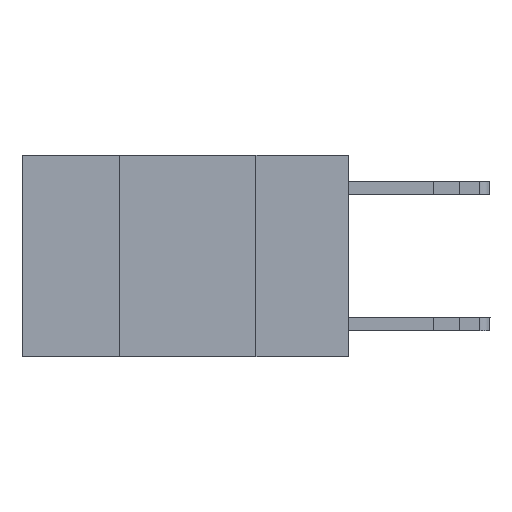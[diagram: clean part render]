
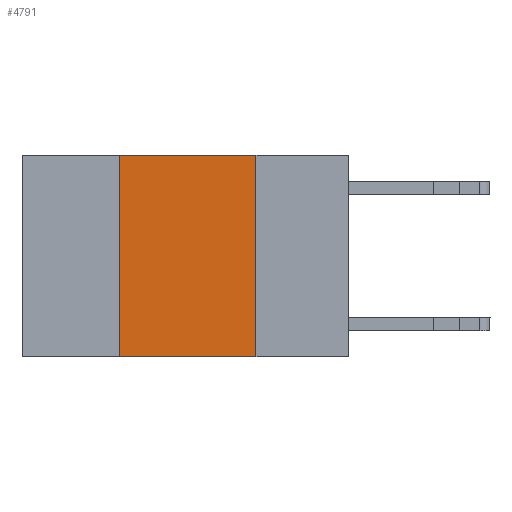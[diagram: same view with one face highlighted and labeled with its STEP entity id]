
A CAD part, left-side view. The second image highlights one B-rep face of the part: STEP entity #4791.
In plain terms, the highlighted planar face has unit normal (-1, 0, 0).
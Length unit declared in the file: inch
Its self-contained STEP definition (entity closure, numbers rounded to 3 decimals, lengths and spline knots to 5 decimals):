
#941 = VECTOR ( 'NONE', #6469, 39.37008 ) ;
#988 = DIRECTION ( 'NONE',  ( 1., 0., 0. ) ) ;
#1052 = LINE ( 'NONE', #8355, #4122 ) ;
#1350 = CARTESIAN_POINT ( 'NONE',  ( 0., 0.17, 0. ) ) ;
#1375 = ORIENTED_EDGE ( 'NONE', *, *, #9001, .T. ) ;
#1661 = LINE ( 'NONE', #10824, #4728 ) ;
#1981 = DIRECTION ( 'NONE',  ( 0., -1., 0. ) ) ;
#3002 = VERTEX_POINT ( 'NONE', #1350 ) ;
#3018 = ORIENTED_EDGE ( 'NONE', *, *, #3946, .F. ) ;
#3277 = VECTOR ( 'NONE', #4234, 39.37008 ) ;
#3498 = VERTEX_POINT ( 'NONE', #16098 ) ;
#3559 = AXIS2_PLACEMENT_3D ( 'NONE', #6138, #988, #9892 ) ;
#3635 = ORIENTED_EDGE ( 'NONE', *, *, #5650, .F. ) ;
#3685 = LINE ( 'NONE', #4189, #3277 ) ;
#3946 = EDGE_CURVE ( 'NONE', #3002, #3498, #1052, .T. ) ;
#4122 = VECTOR ( 'NONE', #10833, 39.37008 ) ;
#4189 = CARTESIAN_POINT ( 'NONE',  ( 0., 0.6, 0. ) ) ;
#4234 = DIRECTION ( 'NONE',  ( 0., -1., 0. ) ) ;
#4728 = VECTOR ( 'NONE', #1981, 39.37008 ) ;
#4791 = ADVANCED_FACE ( 'NONE', ( #7867 ), #7395, .F. ) ;
#5650 = EDGE_CURVE ( 'NONE', #8100, #6380, #11046, .T. ) ;
#6138 = CARTESIAN_POINT ( 'NONE',  ( 0., 0.6, 0. ) ) ;
#6380 = VERTEX_POINT ( 'NONE', #12698 ) ;
#6469 = DIRECTION ( 'NONE',  ( 0., 0., 1. ) ) ;
#6978 = EDGE_LOOP ( 'NONE', ( #3018, #12429, #3635, #1375 ) ) ;
#7395 = PLANE ( 'NONE',  #3559 ) ;
#7867 = FACE_OUTER_BOUND ( 'NONE', #6978, .T. ) ;
#8100 = VERTEX_POINT ( 'NONE', #14008 ) ;
#8355 = CARTESIAN_POINT ( 'NONE',  ( 0., 0.17, 0. ) ) ;
#9001 = EDGE_CURVE ( 'NONE', #8100, #3498, #1661, .T. ) ;
#9892 = DIRECTION ( 'NONE',  ( 0., 0., -1. ) ) ;
#10151 = CARTESIAN_POINT ( 'NONE',  ( 0., 0.42, 0. ) ) ;
#10824 = CARTESIAN_POINT ( 'NONE',  ( 0., 0.6, -0.37 ) ) ;
#10833 = DIRECTION ( 'NONE',  ( 0., 0., -1. ) ) ;
#11046 = LINE ( 'NONE', #10151, #941 ) ;
#12429 = ORIENTED_EDGE ( 'NONE', *, *, #14122, .F. ) ;
#12698 = CARTESIAN_POINT ( 'NONE',  ( 0., 0.42, 0. ) ) ;
#14008 = CARTESIAN_POINT ( 'NONE',  ( 0., 0.42, -0.37 ) ) ;
#14122 = EDGE_CURVE ( 'NONE', #6380, #3002, #3685, .T. ) ;
#16098 = CARTESIAN_POINT ( 'NONE',  ( 0., 0.17, -0.37 ) ) ;
